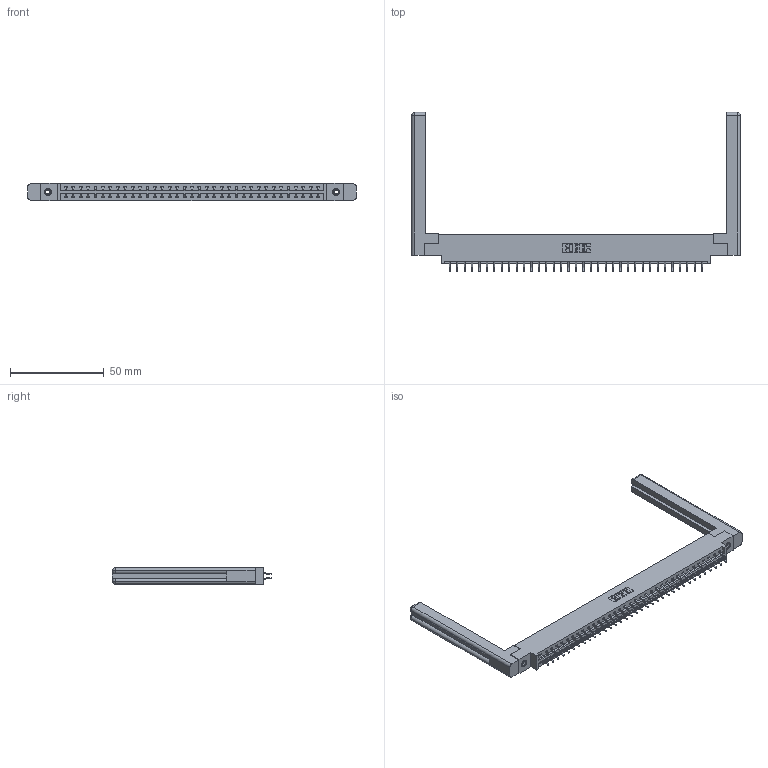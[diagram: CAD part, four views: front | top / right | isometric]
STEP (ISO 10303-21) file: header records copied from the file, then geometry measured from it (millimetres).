
FILE_DESCRIPTION (( 'STEP AP203' ), '1' );
FILE_NAME ('387-070-556-858.STEP', '2019-10-21T23:01:02', ( '' ), ( '' ), 'SwSTEP 2.0', 'SolidWorks 2016', '' );
FILE_SCHEMA (( 'CONFIG_CONTROL_DESIGN' ));
Length unit declared in the file: inch
Products named in the file (5): 345-250-001_345-250-001-102; 345-292-001_556 Tail; 307-220-058; 387-070-556-858; 337 Part_0.170 Offset - 0.156 Dia-TI
Assembly tree (75 placements, depth 2):
  387-070-556-858
    337 Part_0.170 Offset - 0.156 Dia-TI
    345-292-001_556 Tail  x70
    345-250-001_345-250-001-102  x2
    307-220-058  x2
Bounding box: 175.31 x 84.98 x 9.4 mm (x, y, z)
Volume: 25404.5 mm3; surface area: 25658.2 mm2
Topology: 75 solids, 75 shells, 4460 faces, 13207 edges, 8698 vertices
Faces by surface type: plane 3098, cylinder 1338, cone 12, torus 12
Entity records: 31028 total; most frequent: CARTESIAN_POINT 5257, ORIENTED_EDGE 5120, DIRECTION 4488, EDGE_CURVE 2560, LINE 2376, VECTOR 2376, VERTEX_POINT 1698, AXIS2_PLACEMENT_3D 1056
